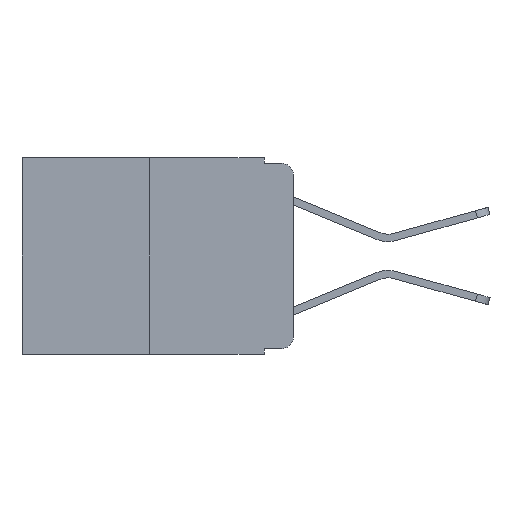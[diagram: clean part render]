
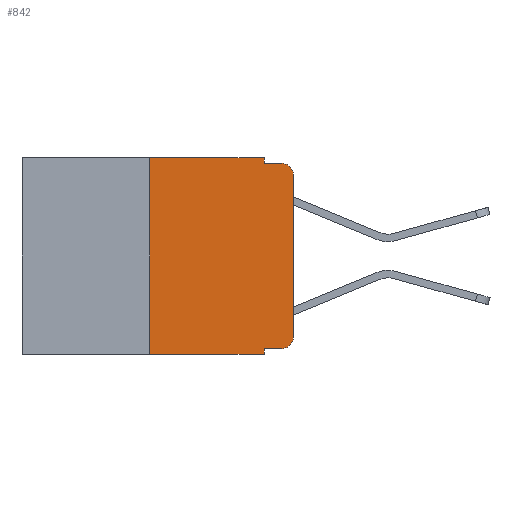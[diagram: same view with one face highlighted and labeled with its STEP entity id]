
A CAD part, left-side view. The second image highlights one B-rep face of the part: STEP entity #842.
In plain terms, the highlighted planar face has unit normal (-1, 0, 0).
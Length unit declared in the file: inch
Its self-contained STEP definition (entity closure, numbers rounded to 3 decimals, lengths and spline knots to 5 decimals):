
#176 = CARTESIAN_POINT ( 'NONE',  ( 0., 0.051, -0.343 ) ) ;
#419 = CARTESIAN_POINT ( 'NONE',  ( 0., 0.051, 0. ) ) ;
#568 = CARTESIAN_POINT ( 'NONE',  ( 0., 0.02, -0.333 ) ) ;
#723 = CARTESIAN_POINT ( 'NONE',  ( 0., 0.473, -0.343 ) ) ;
#835 = DIRECTION ( 'NONE',  ( 0., -1., 0. ) ) ;
#842 = ADVANCED_FACE ( 'NONE', ( #8017 ), #6514, .F. ) ;
#1258 = DIRECTION ( 'NONE',  ( -1., 0., 0. ) ) ;
#1377 = EDGE_CURVE ( 'NONE', #8357, #9841, #7421, .T. ) ;
#1548 = DIRECTION ( 'NONE',  ( 0., -1., 0. ) ) ;
#1758 = CARTESIAN_POINT ( 'NONE',  ( 0., 0., -0.313 ) ) ;
#1922 = VECTOR ( 'NONE', #4483, 39.37008 ) ;
#1979 = DIRECTION ( 'NONE',  ( 0., -1., 0. ) ) ;
#1991 = CARTESIAN_POINT ( 'NONE',  ( 0., 0.051, -0.333 ) ) ;
#2081 = CIRCLE ( 'NONE', #15264, 0.02 ) ;
#2124 = VERTEX_POINT ( 'NONE', #176 ) ;
#2231 = LINE ( 'NONE', #2346, #8432 ) ;
#2346 = CARTESIAN_POINT ( 'NONE',  ( 0., 0.25, 0. ) ) ;
#2472 = VERTEX_POINT ( 'NONE', #3382 ) ;
#2884 = VERTEX_POINT ( 'NONE', #568 ) ;
#2914 = VECTOR ( 'NONE', #1979, 39.37008 ) ;
#3245 = CARTESIAN_POINT ( 'NONE',  ( 0., 0.051, 0. ) ) ;
#3294 = LINE ( 'NONE', #3508, #4252 ) ;
#3336 = EDGE_CURVE ( 'NONE', #2884, #4100, #2081, .T. ) ;
#3382 = CARTESIAN_POINT ( 'NONE',  ( 0., 0.02, -0.01 ) ) ;
#3391 = DIRECTION ( 'NONE',  ( 0., 0., -1. ) ) ;
#3494 = VERTEX_POINT ( 'NONE', #15493 ) ;
#3508 = CARTESIAN_POINT ( 'NONE',  ( 0., 0.051, 0. ) ) ;
#3547 = ORIENTED_EDGE ( 'NONE', *, *, #3336, .T. ) ;
#3554 = EDGE_CURVE ( 'NONE', #13769, #2472, #3629, .T. ) ;
#3629 = CIRCLE ( 'NONE', #4196, 0.02 ) ;
#3669 = EDGE_CURVE ( 'NONE', #4100, #13769, #10006, .T. ) ;
#3859 = DIRECTION ( 'NONE',  ( 0., 0., -1. ) ) ;
#3881 = ORIENTED_EDGE ( 'NONE', *, *, #4298, .T. ) ;
#4100 = VERTEX_POINT ( 'NONE', #1758 ) ;
#4191 = DIRECTION ( 'NONE',  ( 0., 0., 1. ) ) ;
#4196 = AXIS2_PLACEMENT_3D ( 'NONE', #14216, #10807, #7221 ) ;
#4252 = VECTOR ( 'NONE', #3391, 39.37008 ) ;
#4298 = EDGE_CURVE ( 'NONE', #3494, #2124, #5920, .T. ) ;
#4324 = LINE ( 'NONE', #7880, #15727 ) ;
#4476 = CARTESIAN_POINT ( 'NONE',  ( 0., 0.473, 0. ) ) ;
#4483 = DIRECTION ( 'NONE',  ( 0., -1., 0. ) ) ;
#4546 = DIRECTION ( 'NONE',  ( 0., 0., -1. ) ) ;
#5118 = CARTESIAN_POINT ( 'NONE',  ( 0., 0.473, 0. ) ) ;
#5221 = LINE ( 'NONE', #1991, #1922 ) ;
#5544 = ORIENTED_EDGE ( 'NONE', *, *, #6608, .F. ) ;
#5920 = LINE ( 'NONE', #723, #6300 ) ;
#5956 = VECTOR ( 'NONE', #4191, 39.37008 ) ;
#6157 = ORIENTED_EDGE ( 'NONE', *, *, #13520, .T. ) ;
#6300 = VECTOR ( 'NONE', #835, 39.37008 ) ;
#6416 = ORIENTED_EDGE ( 'NONE', *, *, #3669, .T. ) ;
#6514 = PLANE ( 'NONE',  #11386 ) ;
#6608 = EDGE_CURVE ( 'NONE', #9841, #2472, #4324, .T. ) ;
#7221 = DIRECTION ( 'NONE',  ( 0., 0., -1. ) ) ;
#7223 = DIRECTION ( 'NONE',  ( 0., 0., 1. ) ) ;
#7421 = LINE ( 'NONE', #3245, #9522 ) ;
#7814 = EDGE_CURVE ( 'NONE', #14591, #8357, #12369, .T. ) ;
#7880 = CARTESIAN_POINT ( 'NONE',  ( 0., 0.051, -0.01 ) ) ;
#8017 = FACE_OUTER_BOUND ( 'NONE', #13353, .T. ) ;
#8100 = ORIENTED_EDGE ( 'NONE', *, *, #13103, .F. ) ;
#8357 = VERTEX_POINT ( 'NONE', #419 ) ;
#8432 = VECTOR ( 'NONE', #7223, 39.37008 ) ;
#8546 = CARTESIAN_POINT ( 'NONE',  ( 0., 0., -0.03 ) ) ;
#8900 = DIRECTION ( 'NONE',  ( 1., 0., 0. ) ) ;
#9117 = CARTESIAN_POINT ( 'NONE',  ( 0., 0., 0. ) ) ;
#9522 = VECTOR ( 'NONE', #4546, 39.37008 ) ;
#9841 = VERTEX_POINT ( 'NONE', #14214 ) ;
#10006 = LINE ( 'NONE', #9117, #5956 ) ;
#10807 = DIRECTION ( 'NONE',  ( -1., 0., 0. ) ) ;
#10893 = CARTESIAN_POINT ( 'NONE',  ( 0., 0.051, -0.333 ) ) ;
#11386 = AXIS2_PLACEMENT_3D ( 'NONE', #5118, #8900, #12530 ) ;
#12369 = LINE ( 'NONE', #4476, #2914 ) ;
#12381 = ORIENTED_EDGE ( 'NONE', *, *, #1377, .F. ) ;
#12530 = DIRECTION ( 'NONE',  ( 0., 0., -1. ) ) ;
#13103 = EDGE_CURVE ( 'NONE', #14077, #2124, #3294, .T. ) ;
#13353 = EDGE_LOOP ( 'NONE', ( #6416, #15842, #5544, #12381, #15974, #15739, #3881, #8100, #6157, #3547 ) ) ;
#13520 = EDGE_CURVE ( 'NONE', #14077, #2884, #5221, .T. ) ;
#13769 = VERTEX_POINT ( 'NONE', #8546 ) ;
#14077 = VERTEX_POINT ( 'NONE', #10893 ) ;
#14214 = CARTESIAN_POINT ( 'NONE',  ( 0., 0.051, -0.01 ) ) ;
#14216 = CARTESIAN_POINT ( 'NONE',  ( 0., 0.02, -0.03 ) ) ;
#14591 = VERTEX_POINT ( 'NONE', #15356 ) ;
#14842 = CARTESIAN_POINT ( 'NONE',  ( 0., 0.02, -0.313 ) ) ;
#15264 = AXIS2_PLACEMENT_3D ( 'NONE', #14842, #1258, #3859 ) ;
#15356 = CARTESIAN_POINT ( 'NONE',  ( 0., 0.25, 0. ) ) ;
#15493 = CARTESIAN_POINT ( 'NONE',  ( 0., 0.25, -0.343 ) ) ;
#15707 = EDGE_CURVE ( 'NONE', #3494, #14591, #2231, .T. ) ;
#15727 = VECTOR ( 'NONE', #1548, 39.37008 ) ;
#15739 = ORIENTED_EDGE ( 'NONE', *, *, #15707, .F. ) ;
#15842 = ORIENTED_EDGE ( 'NONE', *, *, #3554, .T. ) ;
#15974 = ORIENTED_EDGE ( 'NONE', *, *, #7814, .F. ) ;
